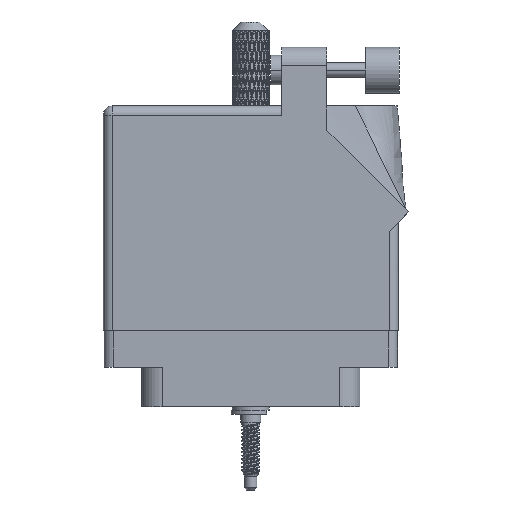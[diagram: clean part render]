
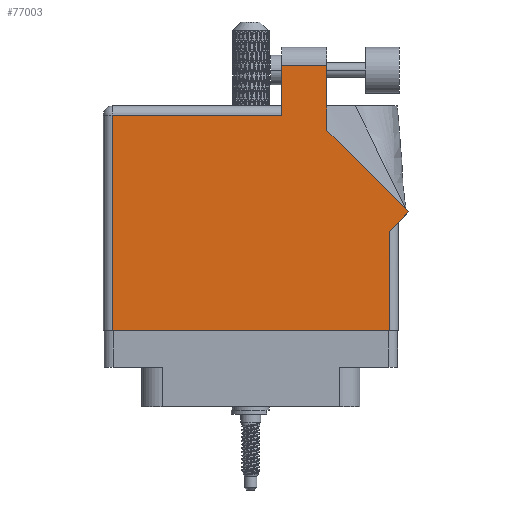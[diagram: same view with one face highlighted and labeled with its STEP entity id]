
A CAD part, front view. The second image highlights one B-rep face of the part: STEP entity #77003.
In plain terms, the highlighted face is planar.
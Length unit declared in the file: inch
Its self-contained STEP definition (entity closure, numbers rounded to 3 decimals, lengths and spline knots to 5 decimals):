
#469 = CARTESIAN_POINT ( 'NONE',  ( 0.212, 1.43, 0.455 ) ) ;
#1288 = VERTEX_POINT ( 'NONE', #94425 ) ;
#3427 = CARTESIAN_POINT ( 'NONE',  ( -1.005, 1.368, 0.455 ) ) ;
#3718 = VECTOR ( 'NONE', #35074, 39.37008 ) ;
#5482 = ORIENTED_EDGE ( 'NONE', *, *, #82019, .T. ) ;
#5556 = VECTOR ( 'NONE', #81046, 39.37008 ) ;
#7349 = AXIS2_PLACEMENT_3D ( 'NONE', #30972, #97888, #32064 ) ;
#7752 = CARTESIAN_POINT ( 'NONE',  ( 0.212, 1.705, 0.455 ) ) ;
#9373 = LINE ( 'NONE', #49595, #5556 ) ;
#10168 = VERTEX_POINT ( 'NONE', #58833 ) ;
#10399 = LINE ( 'NONE', #469, #65260 ) ;
#11114 = FACE_OUTER_BOUND ( 'NONE', #85117, .T. ) ;
#11482 = VECTOR ( 'NONE', #68665, 39.37008 ) ;
#15815 = CARTESIAN_POINT ( 'NONE',  ( -0.943, -0.1, 0.455 ) ) ;
#17878 = VERTEX_POINT ( 'NONE', #7752 ) ;
#17908 = CARTESIAN_POINT ( 'NONE',  ( 1.07571, 0.70771, 0.455 ) ) ;
#19162 = EDGE_CURVE ( 'NONE', #82632, #10168, #67671, .T. ) ;
#21541 = LINE ( 'NONE', #26836, #3718 ) ;
#22963 = EDGE_CURVE ( 'NONE', #105371, #75674, #67379, .T. ) ;
#23111 = CARTESIAN_POINT ( 'NONE',  ( 0.212, 1.705, 0.455 ) ) ;
#24164 = ORIENTED_EDGE ( 'NONE', *, *, #24780, .T. ) ;
#24548 = ORIENTED_EDGE ( 'NONE', *, *, #55994, .T. ) ;
#24780 = EDGE_CURVE ( 'NONE', #10168, #17878, #88910, .T. ) ;
#26536 = VECTOR ( 'NONE', #94860, 39.37008 ) ;
#26836 = CARTESIAN_POINT ( 'NONE',  ( 1.07571, 0.70771, 0.455 ) ) ;
#26946 = VECTOR ( 'NONE', #86974, 39.37008 ) ;
#29044 = CARTESIAN_POINT ( 'NONE',  ( -0.943, -0.1, 0.455 ) ) ;
#29954 = LINE ( 'NONE', #30027, #83715 ) ;
#29990 = VECTOR ( 'NONE', #55596, 39.37008 ) ;
#30027 = CARTESIAN_POINT ( 'NONE',  ( -1.005, -0.1, 0.455 ) ) ;
#30972 = CARTESIAN_POINT ( 'NONE',  ( -1.005, 1.43, 0.455 ) ) ;
#32064 = DIRECTION ( 'NONE',  ( -1., 0., 0. ) ) ;
#34024 = EDGE_CURVE ( 'NONE', #41890, #82632, #21541, .T. ) ;
#35074 = DIRECTION ( 'NONE',  ( -0.707, 0.707, 0. ) ) ;
#41134 = CARTESIAN_POINT ( 'NONE',  ( -0.943, 1.368, 0.455 ) ) ;
#41890 = VERTEX_POINT ( 'NONE', #17908 ) ;
#49595 = CARTESIAN_POINT ( 'NONE',  ( 1.005, 0.637, 0.455 ) ) ;
#52070 = ORIENTED_EDGE ( 'NONE', *, *, #19162, .T. ) ;
#53815 = LINE ( 'NONE', #29044, #26946 ) ;
#55011 = EDGE_CURVE ( 'NONE', #17878, #1288, #10399, .T. ) ;
#55546 = VERTEX_POINT ( 'NONE', #15815 ) ;
#55596 = DIRECTION ( 'NONE',  ( -1., 0., 0. ) ) ;
#55994 = EDGE_CURVE ( 'NONE', #97305, #55546, #53815, .T. ) ;
#56005 = CARTESIAN_POINT ( 'NONE',  ( 0.943, 0.575, 0.455 ) ) ;
#57498 = EDGE_CURVE ( 'NONE', #1288, #97305, #72742, .T. ) ;
#58269 = CARTESIAN_POINT ( 'NONE',  ( 0.943, -0.1, 0.455 ) ) ;
#58833 = CARTESIAN_POINT ( 'NONE',  ( 0.519, 1.705, 0.455 ) ) ;
#61908 = CARTESIAN_POINT ( 'NONE',  ( 0.943, 0.637, 0.455 ) ) ;
#63254 = DIRECTION ( 'NONE',  ( 1., 0., 0. ) ) ;
#65260 = VECTOR ( 'NONE', #65653, 39.37008 ) ;
#65653 = DIRECTION ( 'NONE',  ( 0., -1., 0. ) ) ;
#67379 = LINE ( 'NONE', #61908, #26536 ) ;
#67671 = LINE ( 'NONE', #95753, #80548 ) ;
#68665 = DIRECTION ( 'NONE',  ( -1., 0., 0. ) ) ;
#71021 = DIRECTION ( 'NONE',  ( 0., 1., 0. ) ) ;
#72742 = LINE ( 'NONE', #3427, #11482 ) ;
#75674 = VERTEX_POINT ( 'NONE', #56005 ) ;
#75833 = ORIENTED_EDGE ( 'NONE', *, *, #22963, .T. ) ;
#76577 = CARTESIAN_POINT ( 'NONE',  ( 0.519, 1.26442, 0.455 ) ) ;
#77003 = ADVANCED_FACE ( 'NONE', ( #11114 ), #89595, .F. ) ;
#80126 = EDGE_CURVE ( 'NONE', #55546, #105371, #29954, .T. ) ;
#80548 = VECTOR ( 'NONE', #71021, 39.37008 ) ;
#81046 = DIRECTION ( 'NONE',  ( 0.707, 0.707, 0. ) ) ;
#82019 = EDGE_CURVE ( 'NONE', #75674, #41890, #9373, .T. ) ;
#82632 = VERTEX_POINT ( 'NONE', #76577 ) ;
#83715 = VECTOR ( 'NONE', #63254, 39.37008 ) ;
#85117 = EDGE_LOOP ( 'NONE', ( #52070, #24164, #87772, #98833, #24548, #96591, #75833, #5482, #86809 ) ) ;
#86809 = ORIENTED_EDGE ( 'NONE', *, *, #34024, .T. ) ;
#86974 = DIRECTION ( 'NONE',  ( 0., -1., 0. ) ) ;
#87772 = ORIENTED_EDGE ( 'NONE', *, *, #55011, .T. ) ;
#88910 = LINE ( 'NONE', #23111, #29990 ) ;
#89595 = PLANE ( 'NONE',  #7349 ) ;
#94425 = CARTESIAN_POINT ( 'NONE',  ( 0.212, 1.368, 0.455 ) ) ;
#94860 = DIRECTION ( 'NONE',  ( 0., 1., 0. ) ) ;
#95753 = CARTESIAN_POINT ( 'NONE',  ( 0.519, 1.26442, 0.455 ) ) ;
#96591 = ORIENTED_EDGE ( 'NONE', *, *, #80126, .T. ) ;
#97305 = VERTEX_POINT ( 'NONE', #41134 ) ;
#97888 = DIRECTION ( 'NONE',  ( 0., 0., -1. ) ) ;
#98833 = ORIENTED_EDGE ( 'NONE', *, *, #57498, .T. ) ;
#105371 = VERTEX_POINT ( 'NONE', #58269 ) ;
